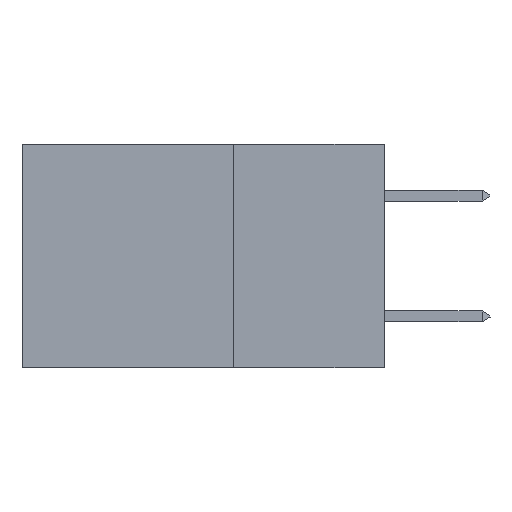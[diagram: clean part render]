
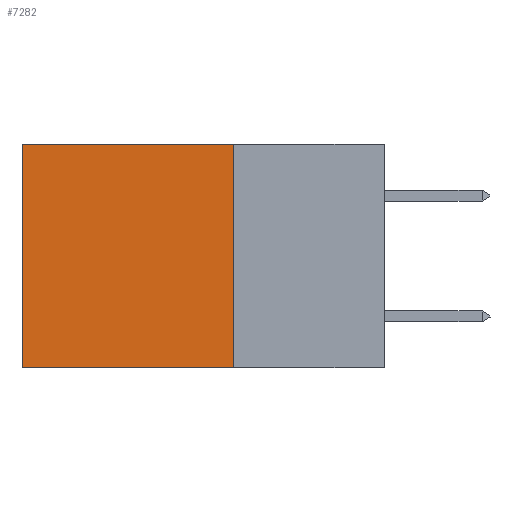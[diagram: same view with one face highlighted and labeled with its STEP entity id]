
A CAD part, left-side view. The second image highlights one B-rep face of the part: STEP entity #7282.
In plain terms, the highlighted planar face has unit normal (-1, 0, 0).
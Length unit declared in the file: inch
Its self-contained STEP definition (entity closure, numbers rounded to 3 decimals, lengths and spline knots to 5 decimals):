
#215 = CARTESIAN_POINT ( 'NONE',  ( 0.2875, 0.6, -0.37 ) ) ;
#708 = EDGE_CURVE ( 'NONE', #18398, #7105, #5439, .T. ) ;
#964 = DIRECTION ( 'NONE',  ( 0., 1., 0. ) ) ;
#1119 = CARTESIAN_POINT ( 'NONE',  ( 0.2875, 0.6, 0. ) ) ;
#1619 = DIRECTION ( 'NONE',  ( 1., 0., 0. ) ) ;
#2187 = VECTOR ( 'NONE', #15766, 39.37008 ) ;
#3544 = LINE ( 'NONE', #9678, #20330 ) ;
#3983 = EDGE_LOOP ( 'NONE', ( #12727, #17820, #17111, #19071 ) ) ;
#4492 = AXIS2_PLACEMENT_3D ( 'NONE', #15386, #1619, #17120 ) ;
#4863 = VECTOR ( 'NONE', #9770, 39.37008 ) ;
#5176 = PLANE ( 'NONE',  #4492 ) ;
#5439 = LINE ( 'NONE', #15612, #2187 ) ;
#5444 = EDGE_CURVE ( 'NONE', #18954, #14819, #3544, .T. ) ;
#5672 = CARTESIAN_POINT ( 'NONE',  ( 0.2875, 0.25, 0. ) ) ;
#6629 = CARTESIAN_POINT ( 'NONE',  ( 0.2875, 0.6, 0. ) ) ;
#7105 = VERTEX_POINT ( 'NONE', #1119 ) ;
#7282 = ADVANCED_FACE ( 'NONE', ( #17908 ), #5176, .F. ) ;
#9678 = CARTESIAN_POINT ( 'NONE',  ( 0.2875, 0.25, -0.37 ) ) ;
#9770 = DIRECTION ( 'NONE',  ( 0., 0., -1. ) ) ;
#11482 = LINE ( 'NONE', #6629, #17926 ) ;
#12727 = ORIENTED_EDGE ( 'NONE', *, *, #17650, .T. ) ;
#13942 = LINE ( 'NONE', #14781, #4863 ) ;
#14781 = CARTESIAN_POINT ( 'NONE',  ( 0.2875, 0.25, 0. ) ) ;
#14819 = VERTEX_POINT ( 'NONE', #215 ) ;
#15386 = CARTESIAN_POINT ( 'NONE',  ( 0.2875, 0.25, 0. ) ) ;
#15612 = CARTESIAN_POINT ( 'NONE',  ( 0.2875, 0.25, 0. ) ) ;
#15766 = DIRECTION ( 'NONE',  ( 0., 1., 0. ) ) ;
#15876 = CARTESIAN_POINT ( 'NONE',  ( 0.2875, 0.25, -0.37 ) ) ;
#17111 = ORIENTED_EDGE ( 'NONE', *, *, #17325, .F. ) ;
#17120 = DIRECTION ( 'NONE',  ( 0., 0., -1. ) ) ;
#17325 = EDGE_CURVE ( 'NONE', #18398, #18954, #13942, .T. ) ;
#17650 = EDGE_CURVE ( 'NONE', #7105, #14819, #11482, .T. ) ;
#17820 = ORIENTED_EDGE ( 'NONE', *, *, #5444, .F. ) ;
#17908 = FACE_OUTER_BOUND ( 'NONE', #3983, .T. ) ;
#17926 = VECTOR ( 'NONE', #20011, 39.37008 ) ;
#18398 = VERTEX_POINT ( 'NONE', #5672 ) ;
#18954 = VERTEX_POINT ( 'NONE', #15876 ) ;
#19071 = ORIENTED_EDGE ( 'NONE', *, *, #708, .T. ) ;
#20011 = DIRECTION ( 'NONE',  ( 0., 0., -1. ) ) ;
#20330 = VECTOR ( 'NONE', #964, 39.37008 ) ;
